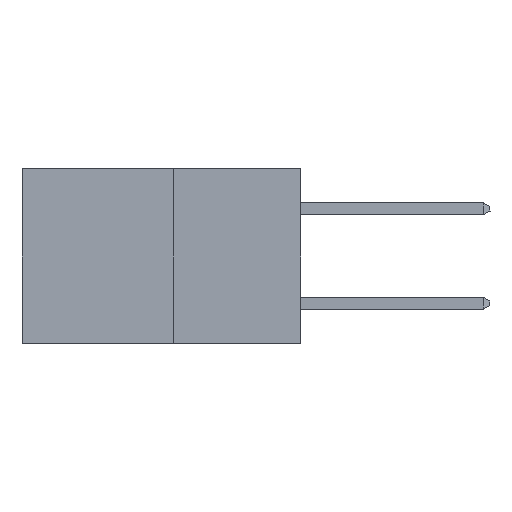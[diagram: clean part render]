
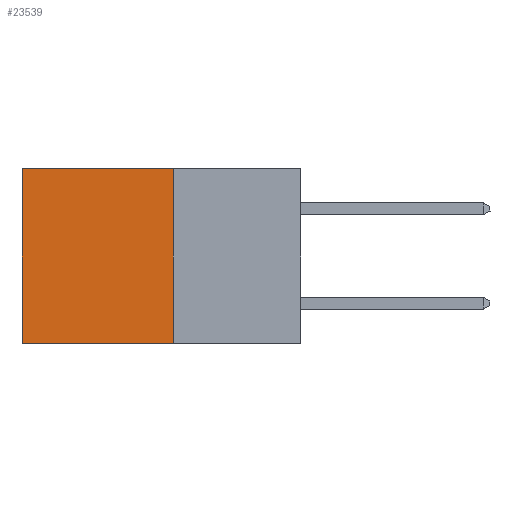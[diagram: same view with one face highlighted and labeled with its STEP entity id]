
A CAD part, left-side view. The second image highlights one B-rep face of the part: STEP entity #23539.
In plain terms, the highlighted planar face has unit normal (-1, 0, 0).
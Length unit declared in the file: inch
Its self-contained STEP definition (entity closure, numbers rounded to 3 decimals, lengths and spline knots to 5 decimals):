
#853 = VECTOR ( 'NONE', #16000, 39.37008 ) ;
#1555 = EDGE_CURVE ( 'NONE', #8526, #5479, #21469, .T. ) ;
#1592 = FACE_OUTER_BOUND ( 'NONE', #25493, .T. ) ;
#2538 = DIRECTION ( 'NONE',  ( 0., 1., 0. ) ) ;
#5479 = VERTEX_POINT ( 'NONE', #12977 ) ;
#7393 = VECTOR ( 'NONE', #2538, 39.37008 ) ;
#7980 = CARTESIAN_POINT ( 'NONE',  ( 0.277, 0.27, -0.37 ) ) ;
#8526 = VERTEX_POINT ( 'NONE', #14690 ) ;
#10247 = VECTOR ( 'NONE', #15621, 39.37008 ) ;
#10555 = ORIENTED_EDGE ( 'NONE', *, *, #18653, .F. ) ;
#11782 = DIRECTION ( 'NONE',  ( 1., 0., 0. ) ) ;
#12372 = LINE ( 'NONE', #7980, #853 ) ;
#12977 = CARTESIAN_POINT ( 'NONE',  ( 0.277, 0.59, -0.37 ) ) ;
#14215 = CARTESIAN_POINT ( 'NONE',  ( 0.277, 0.59, -0.37 ) ) ;
#14654 = DIRECTION ( 'NONE',  ( 0., 0., -1. ) ) ;
#14690 = CARTESIAN_POINT ( 'NONE',  ( 0.277, 0.59, 0. ) ) ;
#14699 = CARTESIAN_POINT ( 'NONE',  ( 0.277, 0.27, 0. ) ) ;
#15621 = DIRECTION ( 'NONE',  ( 0., 0., -1. ) ) ;
#15775 = ORIENTED_EDGE ( 'NONE', *, *, #1555, .T. ) ;
#16000 = DIRECTION ( 'NONE',  ( 0., 1., 0. ) ) ;
#16072 = EDGE_CURVE ( 'NONE', #19028, #20731, #25447, .T. ) ;
#16271 = VECTOR ( 'NONE', #14654, 39.37008 ) ;
#17627 = PLANE ( 'NONE',  #21670 ) ;
#18618 = ORIENTED_EDGE ( 'NONE', *, *, #24200, .T. ) ;
#18653 = EDGE_CURVE ( 'NONE', #20731, #5479, #12372, .T. ) ;
#18963 = ORIENTED_EDGE ( 'NONE', *, *, #16072, .F. ) ;
#19028 = VERTEX_POINT ( 'NONE', #24674 ) ;
#20731 = VERTEX_POINT ( 'NONE', #25916 ) ;
#21469 = LINE ( 'NONE', #14215, #16271 ) ;
#21670 = AXIS2_PLACEMENT_3D ( 'NONE', #23629, #11782, #25632 ) ;
#22608 = LINE ( 'NONE', #14699, #7393 ) ;
#23539 = ADVANCED_FACE ( 'NONE', ( #1592 ), #17627, .F. ) ;
#23629 = CARTESIAN_POINT ( 'NONE',  ( 0.277, 0.27, -0.37 ) ) ;
#24200 = EDGE_CURVE ( 'NONE', #19028, #8526, #22608, .T. ) ;
#24674 = CARTESIAN_POINT ( 'NONE',  ( 0.277, 0.27, 0. ) ) ;
#25447 = LINE ( 'NONE', #25492, #10247 ) ;
#25492 = CARTESIAN_POINT ( 'NONE',  ( 0.277, 0.27, -0.37 ) ) ;
#25493 = EDGE_LOOP ( 'NONE', ( #15775, #10555, #18963, #18618 ) ) ;
#25632 = DIRECTION ( 'NONE',  ( 0., 0., -1. ) ) ;
#25916 = CARTESIAN_POINT ( 'NONE',  ( 0.277, 0.27, -0.37 ) ) ;
